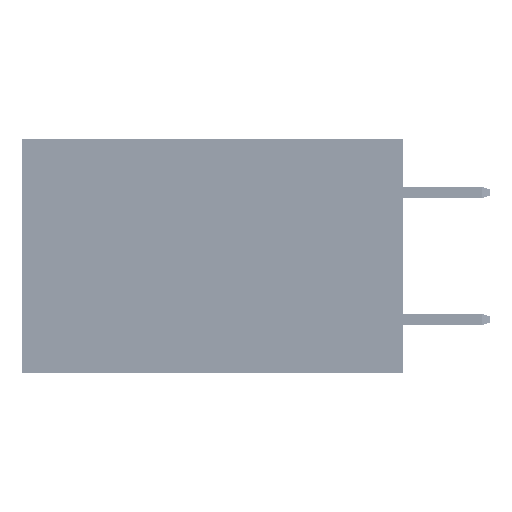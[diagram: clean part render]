
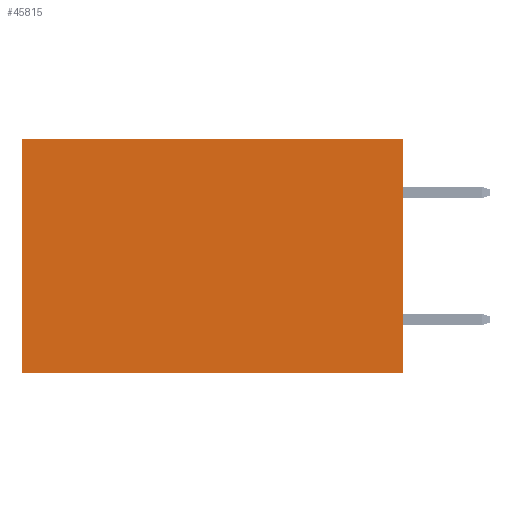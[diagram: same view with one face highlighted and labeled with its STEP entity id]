
A CAD part, left-side view. The second image highlights one B-rep face of the part: STEP entity #45815.
In plain terms, the highlighted planar face has unit normal (-1, 0, 0).
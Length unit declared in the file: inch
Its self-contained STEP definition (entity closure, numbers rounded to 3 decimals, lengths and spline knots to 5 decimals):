
#177 = VECTOR ( 'NONE', #4687, 39.37008 ) ;
#1350 = ORIENTED_EDGE ( 'NONE', *, *, #47694, .F. ) ;
#2418 = CARTESIAN_POINT ( 'NONE',  ( 0.2875, 0.6, -0.37 ) ) ;
#2576 = VECTOR ( 'NONE', #7374, 39.37008 ) ;
#2766 = CARTESIAN_POINT ( 'NONE',  ( 0.2875, 0.6, 0. ) ) ;
#3705 = LINE ( 'NONE', #34672, #4769 ) ;
#4687 = DIRECTION ( 'NONE',  ( 0., 1., 0. ) ) ;
#4769 = VECTOR ( 'NONE', #19418, 39.37008 ) ;
#5590 = ORIENTED_EDGE ( 'NONE', *, *, #32331, .T. ) ;
#5862 = VERTEX_POINT ( 'NONE', #32032 ) ;
#7374 = DIRECTION ( 'NONE',  ( 0., 1., 0. ) ) ;
#7480 = VERTEX_POINT ( 'NONE', #2418 ) ;
#7623 = CARTESIAN_POINT ( 'NONE',  ( 0.2875, 0., -0.37 ) ) ;
#7874 = DIRECTION ( 'NONE',  ( 1., 0., 0. ) ) ;
#7969 = ORIENTED_EDGE ( 'NONE', *, *, #30082, .F. ) ;
#12267 = CARTESIAN_POINT ( 'NONE',  ( 0.2875, 0.6, 0. ) ) ;
#12872 = AXIS2_PLACEMENT_3D ( 'NONE', #38861, #7874, #35516 ) ;
#17312 = LINE ( 'NONE', #48048, #177 ) ;
#19225 = VECTOR ( 'NONE', #20276, 39.37008 ) ;
#19418 = DIRECTION ( 'NONE',  ( 0., 0., -1. ) ) ;
#20276 = DIRECTION ( 'NONE',  ( 0., 0., -1. ) ) ;
#23876 = LINE ( 'NONE', #7623, #2576 ) ;
#25902 = CARTESIAN_POINT ( 'NONE',  ( 0.2875, 0., 0. ) ) ;
#27485 = FACE_OUTER_BOUND ( 'NONE', #50708, .T. ) ;
#30082 = EDGE_CURVE ( 'NONE', #5862, #7480, #23876, .T. ) ;
#32032 = CARTESIAN_POINT ( 'NONE',  ( 0.2875, 0., -0.37 ) ) ;
#32331 = EDGE_CURVE ( 'NONE', #41355, #44359, #17312, .T. ) ;
#34580 = EDGE_CURVE ( 'NONE', #44359, #7480, #39653, .T. ) ;
#34672 = CARTESIAN_POINT ( 'NONE',  ( 0.2875, 0., 0. ) ) ;
#35516 = DIRECTION ( 'NONE',  ( 0., 0., -1. ) ) ;
#36007 = ORIENTED_EDGE ( 'NONE', *, *, #34580, .T. ) ;
#38861 = CARTESIAN_POINT ( 'NONE',  ( 0.2875, 0., 0. ) ) ;
#39653 = LINE ( 'NONE', #12267, #19225 ) ;
#41355 = VERTEX_POINT ( 'NONE', #25902 ) ;
#43270 = PLANE ( 'NONE',  #12872 ) ;
#44359 = VERTEX_POINT ( 'NONE', #2766 ) ;
#45815 = ADVANCED_FACE ( 'NONE', ( #27485 ), #43270, .F. ) ;
#47694 = EDGE_CURVE ( 'NONE', #41355, #5862, #3705, .T. ) ;
#48048 = CARTESIAN_POINT ( 'NONE',  ( 0.2875, 0., 0. ) ) ;
#50708 = EDGE_LOOP ( 'NONE', ( #36007, #7969, #1350, #5590 ) ) ;
